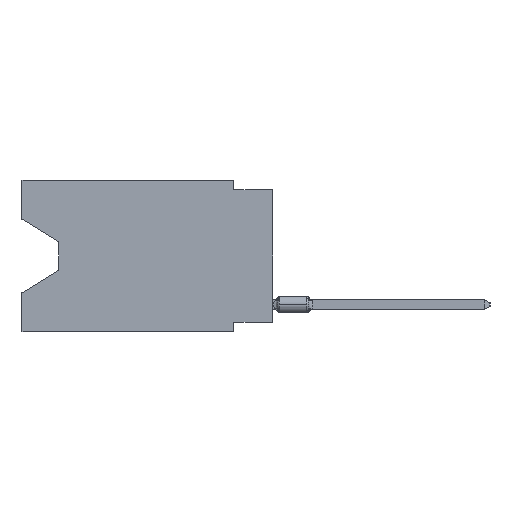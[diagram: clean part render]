
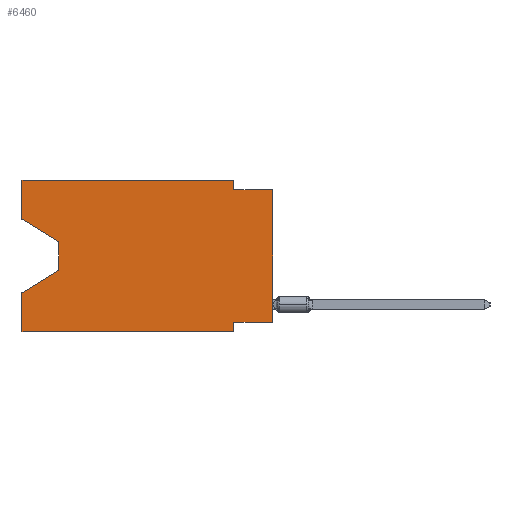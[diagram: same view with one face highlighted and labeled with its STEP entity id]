
A CAD part, left-side view. The second image highlights one B-rep face of the part: STEP entity #6460.
In plain terms, the highlighted planar face has unit normal (-1, 0, 0).
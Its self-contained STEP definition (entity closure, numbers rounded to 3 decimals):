
#379 = ORIENTED_EDGE ( 'NONE', *, *, #17568, .T. ) ;
#2006 = DIRECTION ( 'NONE',  ( 0., 0., 1. ) ) ;
#2728 = ORIENTED_EDGE ( 'NONE', *, *, #57279, .T. ) ;
#3213 = ORIENTED_EDGE ( 'NONE', *, *, #15070, .T. ) ;
#3492 = DIRECTION ( 'NONE',  ( 0., 0., 1. ) ) ;
#4031 = CARTESIAN_POINT ( 'NONE',  ( 0., 2.54, 0. ) ) ;
#4192 = VERTEX_POINT ( 'NONE', #14750 ) ;
#6185 = CARTESIAN_POINT ( 'NONE',  ( 0., 2.54, -9.906 ) ) ;
#6460 = ADVANCED_FACE ( 'NONE', ( #6948 ), #25702, .F. ) ;
#6869 = VECTOR ( 'NONE', #22778, 1000. ) ;
#6918 = LINE ( 'NONE', #52731, #44491 ) ;
#6948 = FACE_OUTER_BOUND ( 'NONE', #53262, .T. ) ;
#7265 = DIRECTION ( 'NONE',  ( 1., 0., 0. ) ) ;
#8415 = DIRECTION ( 'NONE',  ( 0., 0., 1. ) ) ;
#9003 = VECTOR ( 'NONE', #58454, 1000. ) ;
#9057 = CARTESIAN_POINT ( 'NONE',  ( 0., 16.383, -2.546 ) ) ;
#9079 = ORIENTED_EDGE ( 'NONE', *, *, #44138, .F. ) ;
#9653 = CARTESIAN_POINT ( 'NONE',  ( 0., 16.383, -2.546 ) ) ;
#9806 = CARTESIAN_POINT ( 'NONE',  ( 0., 13.97, -5.893 ) ) ;
#10091 = CARTESIAN_POINT ( 'NONE',  ( 0., 2.54, -0.635 ) ) ;
#10872 = DIRECTION ( 'NONE',  ( 0., -0.855, -0.519 ) ) ;
#13374 = DIRECTION ( 'NONE',  ( 0., 0., -1. ) ) ;
#14019 = VECTOR ( 'NONE', #13374, 1000. ) ;
#14058 = CARTESIAN_POINT ( 'NONE',  ( 0., 0., -9.271 ) ) ;
#14421 = ORIENTED_EDGE ( 'NONE', *, *, #45167, .F. ) ;
#14750 = CARTESIAN_POINT ( 'NONE',  ( 0., 13.97, -5.893 ) ) ;
#15070 = EDGE_CURVE ( 'NONE', #18154, #49703, #28020, .T. ) ;
#16363 = ORIENTED_EDGE ( 'NONE', *, *, #45998, .F. ) ;
#16735 = CARTESIAN_POINT ( 'NONE',  ( 0., 2.54, -9.271 ) ) ;
#17568 = EDGE_CURVE ( 'NONE', #57944, #34913, #29627, .T. ) ;
#18154 = VERTEX_POINT ( 'NONE', #39852 ) ;
#22623 = AXIS2_PLACEMENT_3D ( 'NONE', #59460, #7265, #53941 ) ;
#22682 = CARTESIAN_POINT ( 'NONE',  ( 0., 0., -0.635 ) ) ;
#22688 = VECTOR ( 'NONE', #55727, 1000. ) ;
#22778 = DIRECTION ( 'NONE',  ( 0., 0., -1. ) ) ;
#22851 = LINE ( 'NONE', #58783, #56031 ) ;
#23009 = CARTESIAN_POINT ( 'NONE',  ( 0., 16.383, 0. ) ) ;
#23963 = DIRECTION ( 'NONE',  ( 0., 0.855, -0.519 ) ) ;
#24949 = DIRECTION ( 'NONE',  ( 0., 0., -1. ) ) ;
#25532 = EDGE_CURVE ( 'NONE', #25725, #49703, #57489, .T. ) ;
#25702 = PLANE ( 'NONE',  #22623 ) ;
#25725 = VERTEX_POINT ( 'NONE', #16735 ) ;
#25910 = CARTESIAN_POINT ( 'NONE',  ( 0., 0., -9.271 ) ) ;
#27392 = VECTOR ( 'NONE', #46427, 1000. ) ;
#28020 = LINE ( 'NONE', #31717, #27392 ) ;
#28668 = EDGE_CURVE ( 'NONE', #57944, #48107, #45563, .T. ) ;
#29627 = LINE ( 'NONE', #9653, #51199 ) ;
#29926 = LINE ( 'NONE', #25910, #9003 ) ;
#30039 = ORIENTED_EDGE ( 'NONE', *, *, #25532, .F. ) ;
#31717 = CARTESIAN_POINT ( 'NONE',  ( 0., 16.383, -9.906 ) ) ;
#31925 = LINE ( 'NONE', #23009, #59056 ) ;
#32356 = CARTESIAN_POINT ( 'NONE',  ( 0., 2.54, -9.906 ) ) ;
#32572 = VERTEX_POINT ( 'NONE', #10091 ) ;
#33326 = ORIENTED_EDGE ( 'NONE', *, *, #52346, .T. ) ;
#34233 = ORIENTED_EDGE ( 'NONE', *, *, #39567, .F. ) ;
#34632 = VERTEX_POINT ( 'NONE', #54260 ) ;
#34913 = VERTEX_POINT ( 'NONE', #56682 ) ;
#36504 = DIRECTION ( 'NONE',  ( 0., -1., 0. ) ) ;
#37289 = LINE ( 'NONE', #55453, #14019 ) ;
#37757 = LINE ( 'NONE', #9806, #37868 ) ;
#37868 = VECTOR ( 'NONE', #23963, 1000. ) ;
#39280 = EDGE_CURVE ( 'NONE', #32572, #41767, #59729, .T. ) ;
#39567 = EDGE_CURVE ( 'NONE', #52327, #25725, #29926, .T. ) ;
#39852 = CARTESIAN_POINT ( 'NONE',  ( 0., 16.383, -9.906 ) ) ;
#40500 = EDGE_CURVE ( 'NONE', #34913, #4192, #37289, .T. ) ;
#41172 = LINE ( 'NONE', #4031, #6869 ) ;
#41767 = VERTEX_POINT ( 'NONE', #22682 ) ;
#42286 = ORIENTED_EDGE ( 'NONE', *, *, #28668, .F. ) ;
#44138 = EDGE_CURVE ( 'NONE', #34632, #32572, #41172, .T. ) ;
#44491 = VECTOR ( 'NONE', #2006, 1000. ) ;
#44731 = VERTEX_POINT ( 'NONE', #60772 ) ;
#45167 = EDGE_CURVE ( 'NONE', #18154, #44731, #22851, .T. ) ;
#45563 = LINE ( 'NONE', #45855, #47169 ) ;
#45855 = CARTESIAN_POINT ( 'NONE',  ( 0., 16.383, 0. ) ) ;
#45998 = EDGE_CURVE ( 'NONE', #48107, #34632, #31925, .T. ) ;
#46427 = DIRECTION ( 'NONE',  ( 0., -1., 0. ) ) ;
#47169 = VECTOR ( 'NONE', #3492, 1000. ) ;
#47350 = VECTOR ( 'NONE', #24949, 1000. ) ;
#48107 = VERTEX_POINT ( 'NONE', #51106 ) ;
#49703 = VERTEX_POINT ( 'NONE', #32356 ) ;
#51106 = CARTESIAN_POINT ( 'NONE',  ( 0., 16.383, 0. ) ) ;
#51199 = VECTOR ( 'NONE', #10872, 1000. ) ;
#52327 = VERTEX_POINT ( 'NONE', #14058 ) ;
#52346 = EDGE_CURVE ( 'NONE', #52327, #41767, #6918, .T. ) ;
#52731 = CARTESIAN_POINT ( 'NONE',  ( 0., 0., 0. ) ) ;
#53262 = EDGE_LOOP ( 'NONE', ( #379, #56600, #2728, #14421, #3213, #30039, #34233, #33326, #60430, #9079, #16363, #42286 ) ) ;
#53941 = DIRECTION ( 'NONE',  ( 0., 0., -1. ) ) ;
#54260 = CARTESIAN_POINT ( 'NONE',  ( 0., 2.54, 0. ) ) ;
#55132 = CARTESIAN_POINT ( 'NONE',  ( 0., 0., -0.635 ) ) ;
#55453 = CARTESIAN_POINT ( 'NONE',  ( 0., 13.97, -4.013 ) ) ;
#55727 = DIRECTION ( 'NONE',  ( 0., -1., 0. ) ) ;
#56031 = VECTOR ( 'NONE', #8415, 1000. ) ;
#56600 = ORIENTED_EDGE ( 'NONE', *, *, #40500, .T. ) ;
#56682 = CARTESIAN_POINT ( 'NONE',  ( 0., 13.97, -4.013 ) ) ;
#57279 = EDGE_CURVE ( 'NONE', #4192, #44731, #37757, .T. ) ;
#57489 = LINE ( 'NONE', #6185, #47350 ) ;
#57944 = VERTEX_POINT ( 'NONE', #9057 ) ;
#58454 = DIRECTION ( 'NONE',  ( 0., 1., 0. ) ) ;
#58783 = CARTESIAN_POINT ( 'NONE',  ( 0., 16.383, 0. ) ) ;
#59056 = VECTOR ( 'NONE', #36504, 1000. ) ;
#59460 = CARTESIAN_POINT ( 'NONE',  ( 0., 16.383, 0. ) ) ;
#59729 = LINE ( 'NONE', #55132, #22688 ) ;
#60430 = ORIENTED_EDGE ( 'NONE', *, *, #39280, .F. ) ;
#60772 = CARTESIAN_POINT ( 'NONE',  ( 0., 16.383, -7.36 ) ) ;
